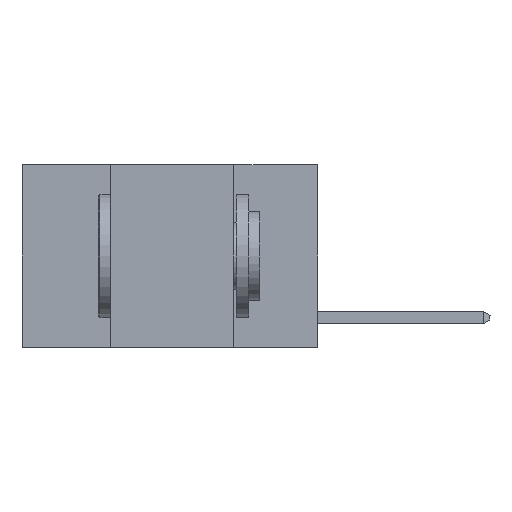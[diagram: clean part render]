
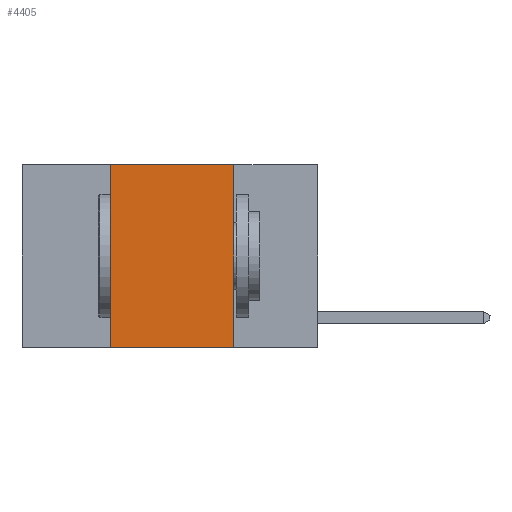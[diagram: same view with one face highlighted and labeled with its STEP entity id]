
A CAD part, left-side view. The second image highlights one B-rep face of the part: STEP entity #4405.
In plain terms, the highlighted planar face has unit normal (-1, 0, 0).
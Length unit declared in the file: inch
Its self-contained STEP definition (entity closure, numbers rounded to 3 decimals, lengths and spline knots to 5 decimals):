
#101 = CARTESIAN_POINT ( 'NONE',  ( 0., 0.17, -0.37 ) ) ;
#368 = ORIENTED_EDGE ( 'NONE', *, *, #4625, .T. ) ;
#769 = CARTESIAN_POINT ( 'NONE',  ( 0., 0.42, 0. ) ) ;
#803 = LINE ( 'NONE', #3631, #823 ) ;
#823 = VECTOR ( 'NONE', #3687, 39.37008 ) ;
#974 = DIRECTION ( 'NONE',  ( 0., 0., -1. ) ) ;
#1086 = CARTESIAN_POINT ( 'NONE',  ( 0., 0.42, -0.37 ) ) ;
#1590 = EDGE_CURVE ( 'NONE', #6385, #6814, #803, .T. ) ;
#1727 = ORIENTED_EDGE ( 'NONE', *, *, #1590, .F. ) ;
#2115 = LINE ( 'NONE', #769, #4521 ) ;
#2832 = CARTESIAN_POINT ( 'NONE',  ( 0., 0.17, 0. ) ) ;
#3110 = CARTESIAN_POINT ( 'NONE',  ( 0., 0.6, 0. ) ) ;
#3163 = VECTOR ( 'NONE', #8636, 39.37008 ) ;
#3205 = ORIENTED_EDGE ( 'NONE', *, *, #8443, .F. ) ;
#3510 = DIRECTION ( 'NONE',  ( 0., 0., 1. ) ) ;
#3540 = VERTEX_POINT ( 'NONE', #1086 ) ;
#3631 = CARTESIAN_POINT ( 'NONE',  ( 0., 0.6, 0. ) ) ;
#3687 = DIRECTION ( 'NONE',  ( 0., -1., 0. ) ) ;
#3987 = PLANE ( 'NONE',  #4646 ) ;
#4245 = VECTOR ( 'NONE', #5783, 39.37008 ) ;
#4348 = ORIENTED_EDGE ( 'NONE', *, *, #6129, .F. ) ;
#4405 = ADVANCED_FACE ( 'NONE', ( #4644 ), #3987, .F. ) ;
#4422 = CARTESIAN_POINT ( 'NONE',  ( 0., 0.17, 0. ) ) ;
#4521 = VECTOR ( 'NONE', #3510, 39.37008 ) ;
#4550 = EDGE_LOOP ( 'NONE', ( #3205, #1727, #4348, #368 ) ) ;
#4625 = EDGE_CURVE ( 'NONE', #3540, #5049, #7180, .T. ) ;
#4644 = FACE_OUTER_BOUND ( 'NONE', #4550, .T. ) ;
#4646 = AXIS2_PLACEMENT_3D ( 'NONE', #3110, #5955, #974 ) ;
#5049 = VERTEX_POINT ( 'NONE', #101 ) ;
#5144 = CARTESIAN_POINT ( 'NONE',  ( 0., 0.6, -0.37 ) ) ;
#5783 = DIRECTION ( 'NONE',  ( 0., 0., -1. ) ) ;
#5955 = DIRECTION ( 'NONE',  ( 1., 0., 0. ) ) ;
#6129 = EDGE_CURVE ( 'NONE', #3540, #6385, #2115, .T. ) ;
#6385 = VERTEX_POINT ( 'NONE', #8104 ) ;
#6814 = VERTEX_POINT ( 'NONE', #4422 ) ;
#7180 = LINE ( 'NONE', #5144, #3163 ) ;
#8104 = CARTESIAN_POINT ( 'NONE',  ( 0., 0.42, 0. ) ) ;
#8443 = EDGE_CURVE ( 'NONE', #6814, #5049, #9319, .T. ) ;
#8636 = DIRECTION ( 'NONE',  ( 0., -1., 0. ) ) ;
#9319 = LINE ( 'NONE', #2832, #4245 ) ;
